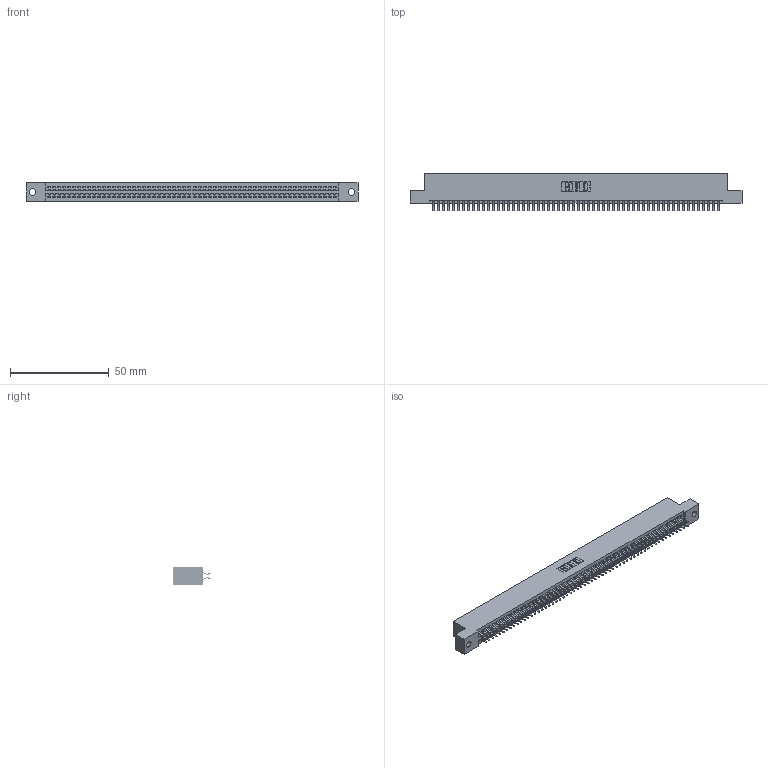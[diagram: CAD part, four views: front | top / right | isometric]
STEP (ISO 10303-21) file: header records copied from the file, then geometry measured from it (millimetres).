
FILE_DESCRIPTION (( 'STEP AP203' ), '1' );
FILE_NAME ('395-116-556-202.STEP', '2018-12-02T02:00:46', ( '' ), ( '' ), 'SwSTEP 2.0', 'SolidWorks 2016', '' );
FILE_SCHEMA (( 'CONFIG_CONTROL_DESIGN' ));
Length unit declared in the file: inch
Products named in the file (3): 345 Part_Flush Mounting Lugs - 0.128 Dia; 345-292-001_556 Tail; 395-116-556-202
Assembly tree (117 placements, depth 2):
  395-116-556-202
    345 Part_Flush Mounting Lugs - 0.128 Dia
    345-292-001_556 Tail  x116
Bounding box: 168.53 x 19.24 x 9.4 mm (x, y, z)
Volume: 16478.3 mm3; surface area: 24293.3 mm2
Topology: 117 solids, 117 shells, 6622 faces, 19713 edges, 12986 vertices
Faces by surface type: plane 4372, cylinder 2250
Entity records: 43577 total; most frequent: CARTESIAN_POINT 7304, ORIENTED_EDGE 7226, DIRECTION 6409, EDGE_CURVE 3613, LINE 3241, VECTOR 3241, VERTEX_POINT 2406, AXIS2_PLACEMENT_3D 1584
